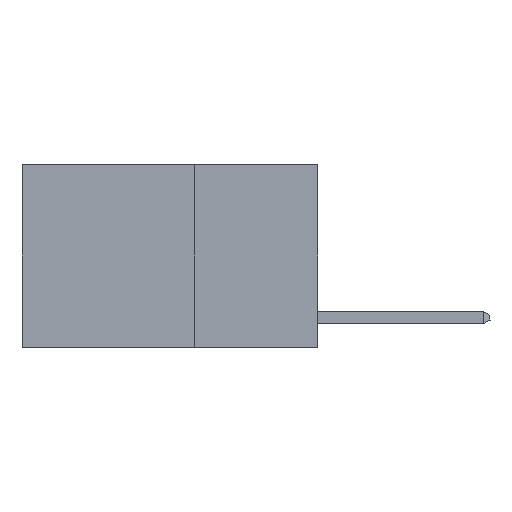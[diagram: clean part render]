
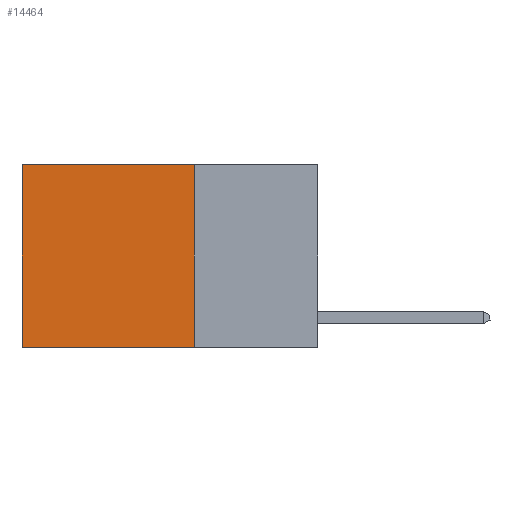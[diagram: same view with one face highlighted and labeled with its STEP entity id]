
A CAD part, left-side view. The second image highlights one B-rep face of the part: STEP entity #14464.
In plain terms, the highlighted planar face has unit normal (-1, 0, 0).
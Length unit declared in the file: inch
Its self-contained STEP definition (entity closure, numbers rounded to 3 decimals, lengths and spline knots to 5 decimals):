
#392 = EDGE_LOOP ( 'NONE', ( #6403, #14633, #16796, #5546 ) ) ;
#910 = EDGE_CURVE ( 'NONE', #4186, #8128, #19109, .T. ) ;
#1413 = VECTOR ( 'NONE', #1441, 39.37008 ) ;
#1441 = DIRECTION ( 'NONE',  ( 0., 0., -1. ) ) ;
#1949 = EDGE_CURVE ( 'NONE', #17902, #8128, #1977, .T. ) ;
#1977 = LINE ( 'NONE', #13770, #17197 ) ;
#2430 = CARTESIAN_POINT ( 'NONE',  ( 0.2625, 0.6, 0. ) ) ;
#3427 = FACE_OUTER_BOUND ( 'NONE', #392, .T. ) ;
#3585 = LINE ( 'NONE', #5346, #14755 ) ;
#4186 = VERTEX_POINT ( 'NONE', #2430 ) ;
#5346 = CARTESIAN_POINT ( 'NONE',  ( 0.2625, 0.25, 0. ) ) ;
#5546 = ORIENTED_EDGE ( 'NONE', *, *, #8030, .T. ) ;
#6403 = ORIENTED_EDGE ( 'NONE', *, *, #910, .T. ) ;
#6885 = CARTESIAN_POINT ( 'NONE',  ( 0.2625, 0.25, -0.37 ) ) ;
#6900 = DIRECTION ( 'NONE',  ( 0., 1., 0. ) ) ;
#7479 = DIRECTION ( 'NONE',  ( 1., 0., 0. ) ) ;
#8030 = EDGE_CURVE ( 'NONE', #17518, #4186, #3585, .T. ) ;
#8128 = VERTEX_POINT ( 'NONE', #14596 ) ;
#11042 = LINE ( 'NONE', #12182, #1413 ) ;
#11887 = PLANE ( 'NONE',  #12829 ) ;
#12046 = CARTESIAN_POINT ( 'NONE',  ( 0.2625, 0.25, 0. ) ) ;
#12182 = CARTESIAN_POINT ( 'NONE',  ( 0.2625, 0.25, 0. ) ) ;
#12829 = AXIS2_PLACEMENT_3D ( 'NONE', #16479, #7479, #17982 ) ;
#13572 = DIRECTION ( 'NONE',  ( 0., 1., 0. ) ) ;
#13770 = CARTESIAN_POINT ( 'NONE',  ( 0.2625, 0.25, -0.37 ) ) ;
#14253 = CARTESIAN_POINT ( 'NONE',  ( 0.2625, 0.6, 0. ) ) ;
#14464 = ADVANCED_FACE ( 'NONE', ( #3427 ), #11887, .F. ) ;
#14596 = CARTESIAN_POINT ( 'NONE',  ( 0.2625, 0.6, -0.37 ) ) ;
#14633 = ORIENTED_EDGE ( 'NONE', *, *, #1949, .F. ) ;
#14755 = VECTOR ( 'NONE', #6900, 39.37008 ) ;
#15322 = DIRECTION ( 'NONE',  ( 0., 0., -1. ) ) ;
#16063 = VECTOR ( 'NONE', #15322, 39.37008 ) ;
#16479 = CARTESIAN_POINT ( 'NONE',  ( 0.2625, 0.25, 0. ) ) ;
#16796 = ORIENTED_EDGE ( 'NONE', *, *, #17568, .F. ) ;
#17197 = VECTOR ( 'NONE', #13572, 39.37008 ) ;
#17518 = VERTEX_POINT ( 'NONE', #12046 ) ;
#17568 = EDGE_CURVE ( 'NONE', #17518, #17902, #11042, .T. ) ;
#17902 = VERTEX_POINT ( 'NONE', #6885 ) ;
#17982 = DIRECTION ( 'NONE',  ( 0., 0., -1. ) ) ;
#19109 = LINE ( 'NONE', #14253, #16063 ) ;
